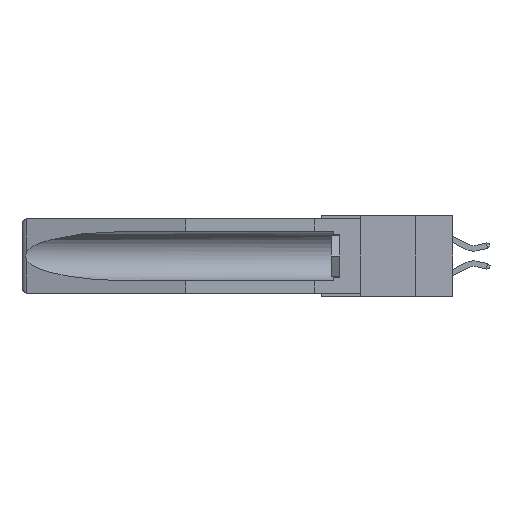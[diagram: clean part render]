
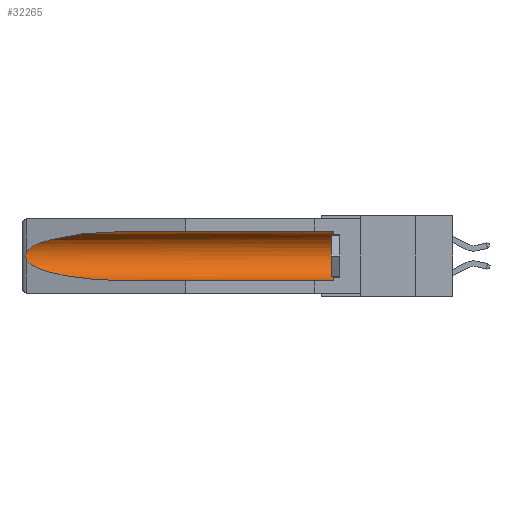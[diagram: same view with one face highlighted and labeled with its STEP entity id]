
A CAD part, left-side view. The second image highlights one B-rep face of the part: STEP entity #32265.
In plain terms, the highlighted cylindrical face has radius 2.857 mm (diameter 5.715 mm), a partial arc.
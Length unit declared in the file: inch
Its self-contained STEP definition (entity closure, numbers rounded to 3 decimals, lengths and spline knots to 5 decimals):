
#320 = CIRCLE ( 'NONE', #1157, 0.1125 ) ;
#479 = EDGE_CURVE ( 'NONE', #17613, #24558, #7932, .T. ) ;
#1018 = DIRECTION ( 'NONE',  ( 0., -1., 0. ) ) ;
#1157 = AXIS2_PLACEMENT_3D ( 'NONE', #3437, #1018, #23842 ) ;
#3180 = CARTESIAN_POINT ( 'NONE',  ( 0.25451, 1.48313, -0.09465 ) ) ;
#3437 = CARTESIAN_POINT ( 'NONE',  ( 0.155, 0.126, -0.1715 ) ) ;
#3491 = DIRECTION ( 'NONE',  ( 0., 1., 0. ) ) ;
#4099 = B_SPLINE_CURVE_WITH_KNOTS ( 'NONE', 3,
 ( #19687, #30222, #5510, #23233, #8040, #28637, #20781, #11030, #10796, #23346 ),
 .UNSPECIFIED., .F., .F.,
 ( 4, 2, 2, 2, 4 ),
 ( 0., 0.00029, 0.00058, 0.00087, 0.00117 ),
 .UNSPECIFIED. ) ;
#4133 = LINE ( 'NONE', #29315, #27893 ) ;
#5004 = EDGE_CURVE ( 'NONE', #30206, #29597, #320, .T. ) ;
#5179 = CARTESIAN_POINT ( 'NONE',  ( 0.155, 0.126, -0.059 ) ) ;
#5297 = ORIENTED_EDGE ( 'NONE', *, *, #23104, .T. ) ;
#5510 = CARTESIAN_POINT ( 'NONE',  ( 0.26654, 1.53092, -0.15636 ) ) ;
#7325 = CARTESIAN_POINT ( 'NONE',  ( 0.21114, 1.30732, -0.284 ) ) ;
#7665 = EDGE_CURVE ( 'NONE', #30206, #24558, #4133, .T. ) ;
#7932 =( BOUNDED_CURVE ( )  B_SPLINE_CURVE ( 3, ( #12323, #19947, #7325, #17509 ),
 .UNSPECIFIED., .F., .F. ) 
 B_SPLINE_CURVE_WITH_KNOTS ( ( 4, 4 ),
 ( 0.1948, 1.5708 ),
 .UNSPECIFIED. ) 
 CURVE ( )  GEOMETRIC_REPRESENTATION_ITEM ( )  RATIONAL_B_SPLINE_CURVE ( ( 1., 0.848, 0.848, 1. ) ) 
 REPRESENTATION_ITEM ( '' )  );
#8040 = CARTESIAN_POINT ( 'NONE',  ( 0.2675, 1.53308, -0.16763 ) ) ;
#9616 = EDGE_LOOP ( 'NONE', ( #16403, #15255, #28105, #14172, #25681, #5297 ) ) ;
#10262 = EDGE_CURVE ( 'NONE', #31200, #12589, #24615, .T. ) ;
#10597 = CARTESIAN_POINT ( 'NONE',  ( 0.155, -0.30754, -0.1715 ) ) ;
#10796 = CARTESIAN_POINT ( 'NONE',  ( 0.26597, 1.5296, -0.19026 ) ) ;
#11030 = CARTESIAN_POINT ( 'NONE',  ( 0.26655, 1.53094, -0.18657 ) ) ;
#12323 = CARTESIAN_POINT ( 'NONE',  ( 0.26537, 1.52718, -0.19328 ) ) ;
#12589 = VERTEX_POINT ( 'NONE', #25191 ) ;
#12820 = EDGE_CURVE ( 'NONE', #12589, #17613, #4099, .T. ) ;
#13071 = DIRECTION ( 'NONE',  ( 0., 0., 1. ) ) ;
#14172 = ORIENTED_EDGE ( 'NONE', *, *, #7665, .F. ) ;
#14569 = CARTESIAN_POINT ( 'NONE',  ( 0.155, 1.07973, -0.059 ) ) ;
#15255 = ORIENTED_EDGE ( 'NONE', *, *, #12820, .T. ) ;
#15500 = AXIS2_PLACEMENT_3D ( 'NONE', #10597, #28338, #13071 ) ;
#16042 = CARTESIAN_POINT ( 'NONE',  ( 0.26537, 1.52718, -0.14972 ) ) ;
#16403 = ORIENTED_EDGE ( 'NONE', *, *, #10262, .T. ) ;
#17509 = CARTESIAN_POINT ( 'NONE',  ( 0.155, 1.07973, -0.284 ) ) ;
#17613 = VERTEX_POINT ( 'NONE', #29037 ) ;
#18224 = CARTESIAN_POINT ( 'NONE',  ( 0.155, 1.07973, -0.059 ) ) ;
#18337 = CARTESIAN_POINT ( 'NONE',  ( 0.21114, 1.30732, -0.059 ) ) ;
#18415 = CARTESIAN_POINT ( 'NONE',  ( 0.155, -0.30754, -0.059 ) ) ;
#19687 = CARTESIAN_POINT ( 'NONE',  ( 0.26537, 1.52718, -0.14972 ) ) ;
#19947 = CARTESIAN_POINT ( 'NONE',  ( 0.25451, 1.48313, -0.24835 ) ) ;
#20781 = CARTESIAN_POINT ( 'NONE',  ( 0.2673, 1.53269, -0.17917 ) ) ;
#23104 = EDGE_CURVE ( 'NONE', #29597, #31200, #30226, .T. ) ;
#23233 = CARTESIAN_POINT ( 'NONE',  ( 0.2673, 1.5327, -0.16383 ) ) ;
#23346 = CARTESIAN_POINT ( 'NONE',  ( 0.26537, 1.52718, -0.19328 ) ) ;
#23530 = DIRECTION ( 'NONE',  ( 0., 1., 0. ) ) ;
#23734 = FACE_OUTER_BOUND ( 'NONE', #9616, .T. ) ;
#23842 = DIRECTION ( 'NONE',  ( 0., 0., 1. ) ) ;
#24558 = VERTEX_POINT ( 'NONE', #28076 ) ;
#24615 =( BOUNDED_CURVE ( )  B_SPLINE_CURVE ( 3, ( #18224, #18337, #3180, #16042 ),
 .UNSPECIFIED., .F., .F. ) 
 B_SPLINE_CURVE_WITH_KNOTS ( ( 4, 4 ),
 ( 4.71239, 6.08839 ),
 .UNSPECIFIED. ) 
 CURVE ( )  GEOMETRIC_REPRESENTATION_ITEM ( )  RATIONAL_B_SPLINE_CURVE ( ( 1., 0.848, 0.848, 1. ) ) 
 REPRESENTATION_ITEM ( '' )  );
#25191 = CARTESIAN_POINT ( 'NONE',  ( 0.26537, 1.52718, -0.14972 ) ) ;
#25681 = ORIENTED_EDGE ( 'NONE', *, *, #5004, .T. ) ;
#27893 = VECTOR ( 'NONE', #3491, 39.37008 ) ;
#28076 = CARTESIAN_POINT ( 'NONE',  ( 0.155, 1.07973, -0.284 ) ) ;
#28105 = ORIENTED_EDGE ( 'NONE', *, *, #479, .T. ) ;
#28338 = DIRECTION ( 'NONE',  ( 0., 1., 0. ) ) ;
#28637 = CARTESIAN_POINT ( 'NONE',  ( 0.2675, 1.53308, -0.17534 ) ) ;
#29037 = CARTESIAN_POINT ( 'NONE',  ( 0.26537, 1.52718, -0.19328 ) ) ;
#29315 = CARTESIAN_POINT ( 'NONE',  ( 0.155, -0.30754, -0.284 ) ) ;
#29597 = VERTEX_POINT ( 'NONE', #5179 ) ;
#30177 = CARTESIAN_POINT ( 'NONE',  ( 0.155, 0.126, -0.284 ) ) ;
#30206 = VERTEX_POINT ( 'NONE', #30177 ) ;
#30222 = CARTESIAN_POINT ( 'NONE',  ( 0.26597, 1.52961, -0.15275 ) ) ;
#30226 = LINE ( 'NONE', #18415, #31034 ) ;
#31034 = VECTOR ( 'NONE', #23530, 39.37008 ) ;
#31200 = VERTEX_POINT ( 'NONE', #14569 ) ;
#32122 = CYLINDRICAL_SURFACE ( 'NONE', #15500, 0.1125 ) ;
#32265 = ADVANCED_FACE ( 'NONE', ( #23734 ), #32122, .F. ) ;
